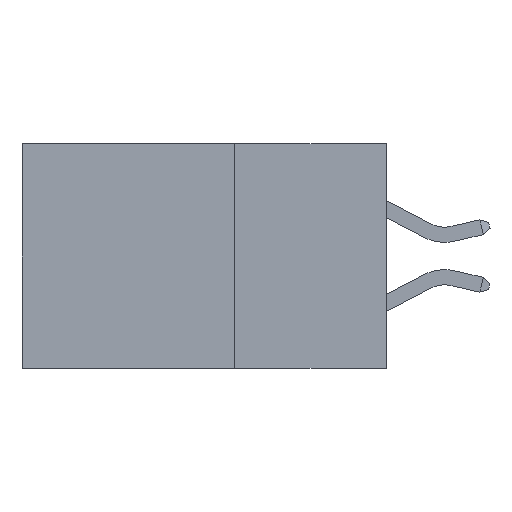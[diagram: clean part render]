
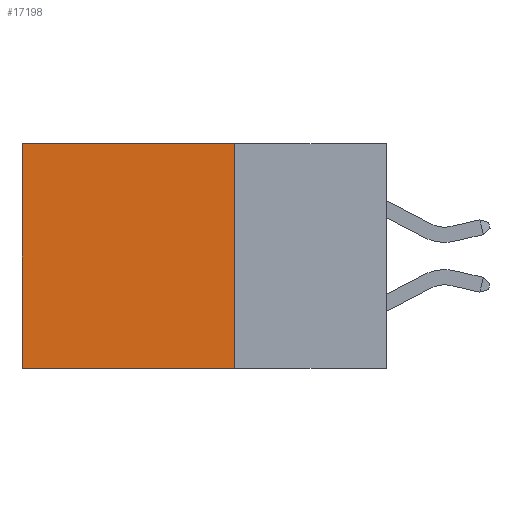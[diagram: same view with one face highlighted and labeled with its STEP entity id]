
A CAD part, left-side view. The second image highlights one B-rep face of the part: STEP entity #17198.
In plain terms, the highlighted planar face has unit normal (-1, 0, 0).
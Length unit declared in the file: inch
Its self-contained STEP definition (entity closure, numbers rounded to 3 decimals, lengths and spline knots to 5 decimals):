
#175 = LINE ( 'NONE', #10863, #6373 ) ;
#235 = CARTESIAN_POINT ( 'NONE',  ( 0.2615, 0.25, -0.37 ) ) ;
#2085 = CARTESIAN_POINT ( 'NONE',  ( 0.2615, 0.25, -0.37 ) ) ;
#2992 = VERTEX_POINT ( 'NONE', #7302 ) ;
#3413 = ORIENTED_EDGE ( 'NONE', *, *, #12980, .F. ) ;
#6077 = CARTESIAN_POINT ( 'NONE',  ( 0.2615, 0.25, 0. ) ) ;
#6084 = EDGE_CURVE ( 'NONE', #16731, #2992, #175, .T. ) ;
#6125 = DIRECTION ( 'NONE',  ( 0., 0., -1. ) ) ;
#6373 = VECTOR ( 'NONE', #10966, 39.37008 ) ;
#7047 = EDGE_LOOP ( 'NONE', ( #7671, #12624, #3413, #10195 ) ) ;
#7302 = CARTESIAN_POINT ( 'NONE',  ( 0.2615, 0.6, -0.37 ) ) ;
#7419 = EDGE_CURVE ( 'NONE', #13178, #2992, #17362, .T. ) ;
#7671 = ORIENTED_EDGE ( 'NONE', *, *, #6084, .T. ) ;
#8283 = DIRECTION ( 'NONE',  ( 0., 1., 0. ) ) ;
#8920 = VECTOR ( 'NONE', #15989, 39.37008 ) ;
#10195 = ORIENTED_EDGE ( 'NONE', *, *, #12295, .T. ) ;
#10767 = CARTESIAN_POINT ( 'NONE',  ( 0.2615, 0.25, -0.37 ) ) ;
#10863 = CARTESIAN_POINT ( 'NONE',  ( 0.2615, 0.6, -0.37 ) ) ;
#10966 = DIRECTION ( 'NONE',  ( 0., 0., -1. ) ) ;
#11476 = CARTESIAN_POINT ( 'NONE',  ( 0.2615, 0.6, 0. ) ) ;
#12229 = FACE_OUTER_BOUND ( 'NONE', #7047, .T. ) ;
#12295 = EDGE_CURVE ( 'NONE', #16215, #16731, #17576, .T. ) ;
#12624 = ORIENTED_EDGE ( 'NONE', *, *, #7419, .F. ) ;
#12980 = EDGE_CURVE ( 'NONE', #16215, #13178, #19557, .T. ) ;
#13178 = VERTEX_POINT ( 'NONE', #10767 ) ;
#13567 = DIRECTION ( 'NONE',  ( 0., 0., -1. ) ) ;
#13631 = DIRECTION ( 'NONE',  ( 1., 0., 0. ) ) ;
#13772 = CARTESIAN_POINT ( 'NONE',  ( 0.2615, 0.25, -0.37 ) ) ;
#15989 = DIRECTION ( 'NONE',  ( 0., 1., 0. ) ) ;
#16215 = VERTEX_POINT ( 'NONE', #6077 ) ;
#16369 = AXIS2_PLACEMENT_3D ( 'NONE', #235, #13631, #6125 ) ;
#16608 = PLANE ( 'NONE',  #16369 ) ;
#16731 = VERTEX_POINT ( 'NONE', #11476 ) ;
#17099 = VECTOR ( 'NONE', #8283, 39.37008 ) ;
#17198 = ADVANCED_FACE ( 'NONE', ( #12229 ), #16608, .F. ) ;
#17362 = LINE ( 'NONE', #2085, #17099 ) ;
#17576 = LINE ( 'NONE', #19077, #8920 ) ;
#18475 = VECTOR ( 'NONE', #13567, 39.37008 ) ;
#19077 = CARTESIAN_POINT ( 'NONE',  ( 0.2615, 0.25, 0. ) ) ;
#19557 = LINE ( 'NONE', #13772, #18475 ) ;
